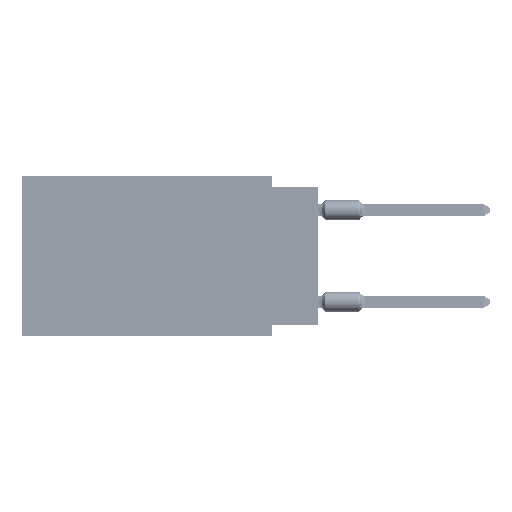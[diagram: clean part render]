
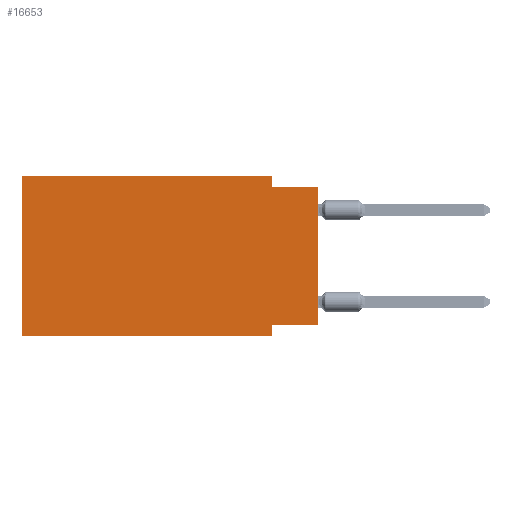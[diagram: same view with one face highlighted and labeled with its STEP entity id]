
A CAD part, left-side view. The second image highlights one B-rep face of the part: STEP entity #16653.
In plain terms, the highlighted planar face has unit normal (-1, 0, 0).
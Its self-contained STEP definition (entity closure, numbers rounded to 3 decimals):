
#3016 = EDGE_CURVE ( 'NONE', #77649, #90165, #71593, .T. ) ;
#3438 = VERTEX_POINT ( 'NONE', #89540 ) ;
#3993 = LINE ( 'NONE', #60979, #30553 ) ;
#7449 = LINE ( 'NONE', #35961, #23070 ) ;
#7667 = DIRECTION ( 'NONE',  ( 0., -1., 0. ) ) ;
#9032 = LINE ( 'NONE', #37540, #58596 ) ;
#10900 = AXIS2_PLACEMENT_3D ( 'NONE', #23502, #46809, #73944 ) ;
#11758 = VECTOR ( 'NONE', #7667, 1000. ) ;
#13085 = CARTESIAN_POINT ( 'NONE',  ( 0., 0., 0. ) ) ;
#16653 = ADVANCED_FACE ( 'NONE', ( #75307 ), #38896, .F. ) ;
#17163 = ORIENTED_EDGE ( 'NONE', *, *, #55014, .F. ) ;
#18607 = DIRECTION ( 'NONE',  ( 0., 0., 1. ) ) ;
#20313 = DIRECTION ( 'NONE',  ( 0., -1., 0. ) ) ;
#22064 = CARTESIAN_POINT ( 'NONE',  ( 0., 2.54, -0.635 ) ) ;
#23070 = VECTOR ( 'NONE', #71909, 1000. ) ;
#23295 = EDGE_CURVE ( 'NONE', #3438, #59873, #78486, .T. ) ;
#23502 = CARTESIAN_POINT ( 'NONE',  ( 0., 16.383, 0. ) ) ;
#28038 = DIRECTION ( 'NONE',  ( 0., 0., 1. ) ) ;
#30553 = VECTOR ( 'NONE', #20313, 1000. ) ;
#35464 = VECTOR ( 'NONE', #28038, 1000. ) ;
#35961 = CARTESIAN_POINT ( 'NONE',  ( 0., 0., -0.635 ) ) ;
#36008 = VERTEX_POINT ( 'NONE', #46285 ) ;
#37146 = DIRECTION ( 'NONE',  ( 0., 1., 0. ) ) ;
#37540 = CARTESIAN_POINT ( 'NONE',  ( 0., 2.54, -8.89 ) ) ;
#38896 = PLANE ( 'NONE',  #10900 ) ;
#42858 = VECTOR ( 'NONE', #37146, 1000. ) ;
#45167 = EDGE_CURVE ( 'NONE', #69998, #80115, #76509, .T. ) ;
#46285 = CARTESIAN_POINT ( 'NONE',  ( 0., 2.54, -8.89 ) ) ;
#46314 = EDGE_CURVE ( 'NONE', #3438, #76973, #69873, .T. ) ;
#46809 = DIRECTION ( 'NONE',  ( 1., 0., 0. ) ) ;
#48769 = CARTESIAN_POINT ( 'NONE',  ( 0., 16.383, -8.89 ) ) ;
#54546 = ORIENTED_EDGE ( 'NONE', *, *, #71431, .F. ) ;
#55014 = EDGE_CURVE ( 'NONE', #76973, #36008, #9032, .T. ) ;
#56407 = EDGE_CURVE ( 'NONE', #69998, #36008, #3993, .T. ) ;
#56867 = EDGE_CURVE ( 'NONE', #90165, #59873, #7449, .T. ) ;
#57642 = LINE ( 'NONE', #71676, #11758 ) ;
#58596 = VECTOR ( 'NONE', #59012, 1000. ) ;
#59012 = DIRECTION ( 'NONE',  ( 0., 0., -1. ) ) ;
#59873 = VERTEX_POINT ( 'NONE', #67534 ) ;
#60599 = CARTESIAN_POINT ( 'NONE',  ( 0., 16.383, 0. ) ) ;
#60979 = CARTESIAN_POINT ( 'NONE',  ( 0., 16.383, -8.89 ) ) ;
#62101 = ORIENTED_EDGE ( 'NONE', *, *, #46314, .F. ) ;
#62863 = CARTESIAN_POINT ( 'NONE',  ( 0., 0., -8.255 ) ) ;
#67534 = CARTESIAN_POINT ( 'NONE',  ( 0., 0., -0.635 ) ) ;
#68581 = CARTESIAN_POINT ( 'NONE',  ( 0., 16.383, 0. ) ) ;
#68727 = ORIENTED_EDGE ( 'NONE', *, *, #3016, .F. ) ;
#69873 = LINE ( 'NONE', #62863, #42858 ) ;
#69998 = VERTEX_POINT ( 'NONE', #48769 ) ;
#70333 = CARTESIAN_POINT ( 'NONE',  ( 0., 2.54, 0. ) ) ;
#70995 = ORIENTED_EDGE ( 'NONE', *, *, #45167, .F. ) ;
#71431 = EDGE_CURVE ( 'NONE', #80115, #77649, #57642, .T. ) ;
#71593 = LINE ( 'NONE', #72046, #82174 ) ;
#71676 = CARTESIAN_POINT ( 'NONE',  ( 0., 16.383, 0. ) ) ;
#71909 = DIRECTION ( 'NONE',  ( 0., -1., 0. ) ) ;
#72046 = CARTESIAN_POINT ( 'NONE',  ( 0., 2.54, 0. ) ) ;
#73944 = DIRECTION ( 'NONE',  ( 0., 0., -1. ) ) ;
#75307 = FACE_OUTER_BOUND ( 'NONE', #89704, .T. ) ;
#75539 = VECTOR ( 'NONE', #18607, 1000. ) ;
#76509 = LINE ( 'NONE', #68581, #75539 ) ;
#76973 = VERTEX_POINT ( 'NONE', #87130 ) ;
#77649 = VERTEX_POINT ( 'NONE', #70333 ) ;
#78486 = LINE ( 'NONE', #13085, #35464 ) ;
#79531 = DIRECTION ( 'NONE',  ( 0., 0., -1. ) ) ;
#80115 = VERTEX_POINT ( 'NONE', #60599 ) ;
#82174 = VECTOR ( 'NONE', #79531, 1000. ) ;
#83249 = ORIENTED_EDGE ( 'NONE', *, *, #23295, .T. ) ;
#86249 = ORIENTED_EDGE ( 'NONE', *, *, #56407, .T. ) ;
#87130 = CARTESIAN_POINT ( 'NONE',  ( 0., 2.54, -8.255 ) ) ;
#87219 = ORIENTED_EDGE ( 'NONE', *, *, #56867, .F. ) ;
#89540 = CARTESIAN_POINT ( 'NONE',  ( 0., 0., -8.255 ) ) ;
#89704 = EDGE_LOOP ( 'NONE', ( #83249, #87219, #68727, #54546, #70995, #86249, #17163, #62101 ) ) ;
#90165 = VERTEX_POINT ( 'NONE', #22064 ) ;
